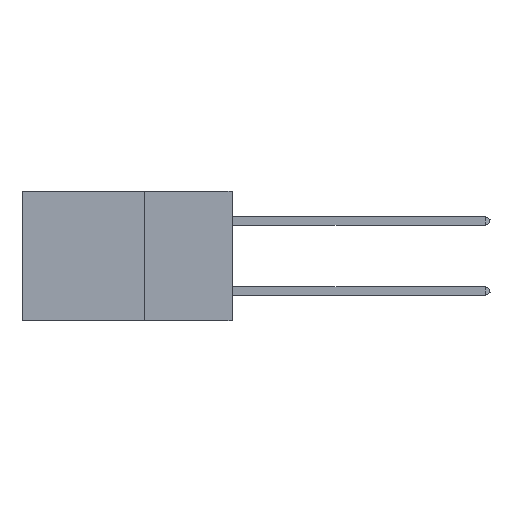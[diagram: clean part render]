
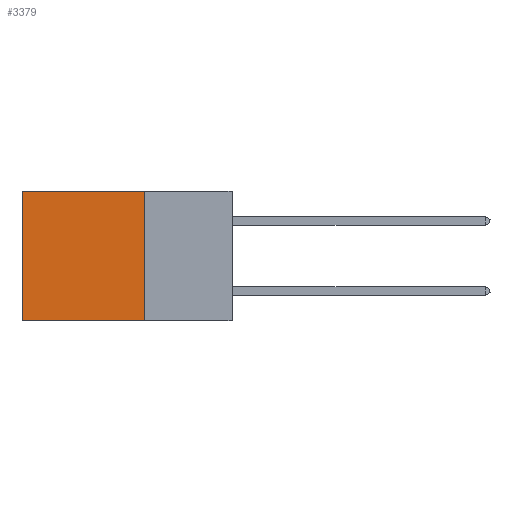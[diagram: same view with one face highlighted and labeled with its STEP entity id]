
A CAD part, left-side view. The second image highlights one B-rep face of the part: STEP entity #3379.
In plain terms, the highlighted planar face has unit normal (-1, 0, 0).
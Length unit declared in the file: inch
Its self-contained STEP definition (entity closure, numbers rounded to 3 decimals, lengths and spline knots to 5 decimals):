
#560 = LINE ( 'NONE', #30289, #25648 ) ;
#916 = FACE_OUTER_BOUND ( 'NONE', #15358, .T. ) ;
#2935 = PLANE ( 'NONE',  #7532 ) ;
#3224 = EDGE_CURVE ( 'NONE', #9631, #13232, #5473, .T. ) ;
#3379 = ADVANCED_FACE ( 'NONE', ( #916 ), #2935, .F. ) ;
#5225 = CARTESIAN_POINT ( 'NONE',  ( 0.2875, 0.6, -0.37 ) ) ;
#5473 = LINE ( 'NONE', #20069, #34349 ) ;
#6750 = CARTESIAN_POINT ( 'NONE',  ( 0.2875, 0.6, 0. ) ) ;
#7532 = AXIS2_PLACEMENT_3D ( 'NONE', #14593, #17141, #25006 ) ;
#7691 = VECTOR ( 'NONE', #18735, 39.37008 ) ;
#9631 = VERTEX_POINT ( 'NONE', #23904 ) ;
#13232 = VERTEX_POINT ( 'NONE', #32277 ) ;
#14593 = CARTESIAN_POINT ( 'NONE',  ( 0.2875, 0.25, 0. ) ) ;
#15358 = EDGE_LOOP ( 'NONE', ( #21844, #27556, #16893, #17334 ) ) ;
#15639 = CARTESIAN_POINT ( 'NONE',  ( 0.2875, 0.6, 0. ) ) ;
#16893 = ORIENTED_EDGE ( 'NONE', *, *, #3224, .F. ) ;
#17129 = VECTOR ( 'NONE', #23707, 39.37008 ) ;
#17141 = DIRECTION ( 'NONE',  ( 1., 0., 0. ) ) ;
#17334 = ORIENTED_EDGE ( 'NONE', *, *, #25716, .T. ) ;
#18735 = DIRECTION ( 'NONE',  ( 0., 1., 0. ) ) ;
#18979 = CARTESIAN_POINT ( 'NONE',  ( 0.2875, 0.25, 0. ) ) ;
#20031 = VERTEX_POINT ( 'NONE', #5225 ) ;
#20069 = CARTESIAN_POINT ( 'NONE',  ( 0.2875, 0.25, 0. ) ) ;
#21844 = ORIENTED_EDGE ( 'NONE', *, *, #32813, .T. ) ;
#22168 = LINE ( 'NONE', #15639, #17129 ) ;
#22527 = VERTEX_POINT ( 'NONE', #6750 ) ;
#23707 = DIRECTION ( 'NONE',  ( 0., 0., -1. ) ) ;
#23904 = CARTESIAN_POINT ( 'NONE',  ( 0.2875, 0.25, 0. ) ) ;
#25006 = DIRECTION ( 'NONE',  ( 0., 0., -1. ) ) ;
#25648 = VECTOR ( 'NONE', #32744, 39.37008 ) ;
#25716 = EDGE_CURVE ( 'NONE', #9631, #22527, #30291, .T. ) ;
#27556 = ORIENTED_EDGE ( 'NONE', *, *, #29923, .F. ) ;
#29923 = EDGE_CURVE ( 'NONE', #13232, #20031, #560, .T. ) ;
#30289 = CARTESIAN_POINT ( 'NONE',  ( 0.2875, 0.25, -0.37 ) ) ;
#30291 = LINE ( 'NONE', #18979, #7691 ) ;
#32277 = CARTESIAN_POINT ( 'NONE',  ( 0.2875, 0.25, -0.37 ) ) ;
#32744 = DIRECTION ( 'NONE',  ( 0., 1., 0. ) ) ;
#32813 = EDGE_CURVE ( 'NONE', #22527, #20031, #22168, .T. ) ;
#33809 = DIRECTION ( 'NONE',  ( 0., 0., -1. ) ) ;
#34349 = VECTOR ( 'NONE', #33809, 39.37008 ) ;
